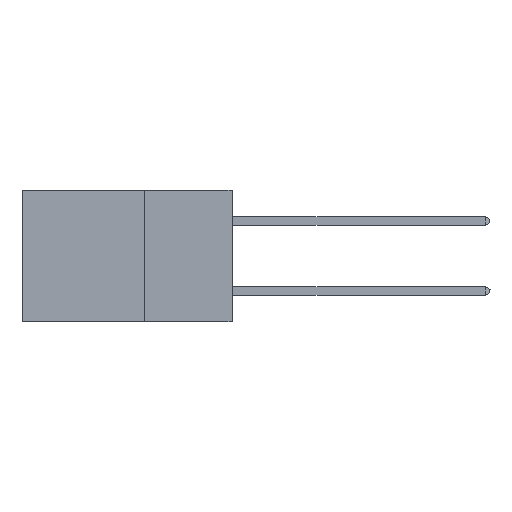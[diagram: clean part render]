
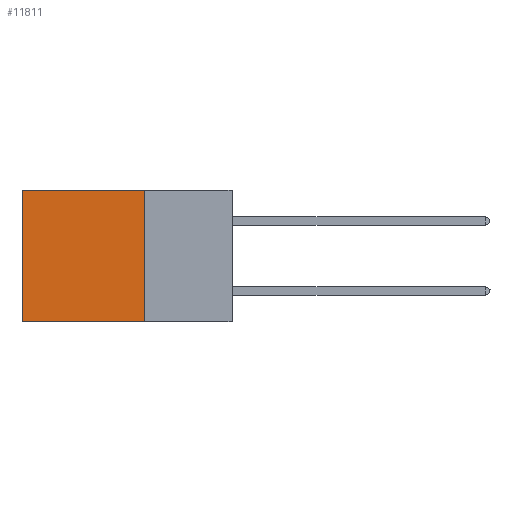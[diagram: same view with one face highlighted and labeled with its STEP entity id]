
A CAD part, left-side view. The second image highlights one B-rep face of the part: STEP entity #11811.
In plain terms, the highlighted planar face has unit normal (-1, 0, 0).
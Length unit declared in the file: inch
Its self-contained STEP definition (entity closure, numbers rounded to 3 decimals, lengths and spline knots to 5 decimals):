
#25 = DIRECTION ( 'NONE',  ( 0., 0., -1. ) ) ;
#86 = VERTEX_POINT ( 'NONE', #4622 ) ;
#295 = CARTESIAN_POINT ( 'NONE',  ( 0.2875, 0.25, -0.375 ) ) ;
#703 = DIRECTION ( 'NONE',  ( 0., 1., 0. ) ) ;
#1635 = VECTOR ( 'NONE', #703, 39.37008 ) ;
#1808 = ORIENTED_EDGE ( 'NONE', *, *, #14286, .T. ) ;
#2143 = CARTESIAN_POINT ( 'NONE',  ( 0.2875, 0.6, 0. ) ) ;
#2548 = EDGE_CURVE ( 'NONE', #7962, #11340, #5017, .T. ) ;
#2631 = CARTESIAN_POINT ( 'NONE',  ( 0.2875, 0.25, -0.375 ) ) ;
#2934 = VECTOR ( 'NONE', #15367, 39.37008 ) ;
#3128 = ORIENTED_EDGE ( 'NONE', *, *, #13593, .T. ) ;
#3248 = FACE_OUTER_BOUND ( 'NONE', #14098, .T. ) ;
#3622 = CARTESIAN_POINT ( 'NONE',  ( 0.2875, 0.25, 0. ) ) ;
#3679 = VECTOR ( 'NONE', #5118, 39.37008 ) ;
#4008 = CARTESIAN_POINT ( 'NONE',  ( 0.2875, 0.25, -0.375 ) ) ;
#4221 = CARTESIAN_POINT ( 'NONE',  ( 0.2875, 0.25, -0.375 ) ) ;
#4622 = CARTESIAN_POINT ( 'NONE',  ( 0.2875, 0.6, -0.375 ) ) ;
#4943 = DIRECTION ( 'NONE',  ( 1., 0., 0. ) ) ;
#5017 = LINE ( 'NONE', #295, #3679 ) ;
#5118 = DIRECTION ( 'NONE',  ( 0., 0., -1. ) ) ;
#5819 = DIRECTION ( 'NONE',  ( 0., 1., 0. ) ) ;
#6171 = LINE ( 'NONE', #6842, #2934 ) ;
#6189 = VERTEX_POINT ( 'NONE', #2143 ) ;
#6842 = CARTESIAN_POINT ( 'NONE',  ( 0.2875, 0.6, -0.375 ) ) ;
#7879 = LINE ( 'NONE', #4221, #1635 ) ;
#7962 = VERTEX_POINT ( 'NONE', #3622 ) ;
#8276 = VECTOR ( 'NONE', #5819, 39.37008 ) ;
#10362 = AXIS2_PLACEMENT_3D ( 'NONE', #2631, #4943, #25 ) ;
#11340 = VERTEX_POINT ( 'NONE', #4008 ) ;
#11440 = ORIENTED_EDGE ( 'NONE', *, *, #14139, .F. ) ;
#11479 = LINE ( 'NONE', #13149, #8276 ) ;
#11811 = ADVANCED_FACE ( 'NONE', ( #3248 ), #14582, .F. ) ;
#12282 = ORIENTED_EDGE ( 'NONE', *, *, #2548, .F. ) ;
#13149 = CARTESIAN_POINT ( 'NONE',  ( 0.2875, 0.25, 0. ) ) ;
#13593 = EDGE_CURVE ( 'NONE', #6189, #86, #6171, .T. ) ;
#14098 = EDGE_LOOP ( 'NONE', ( #3128, #11440, #12282, #1808 ) ) ;
#14139 = EDGE_CURVE ( 'NONE', #11340, #86, #7879, .T. ) ;
#14286 = EDGE_CURVE ( 'NONE', #7962, #6189, #11479, .T. ) ;
#14582 = PLANE ( 'NONE',  #10362 ) ;
#15367 = DIRECTION ( 'NONE',  ( 0., 0., -1. ) ) ;
